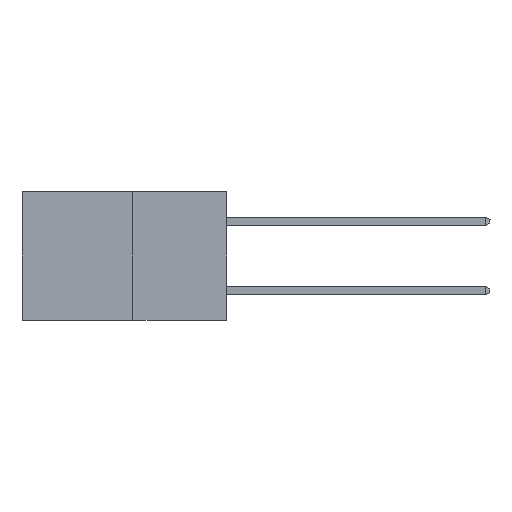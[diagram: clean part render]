
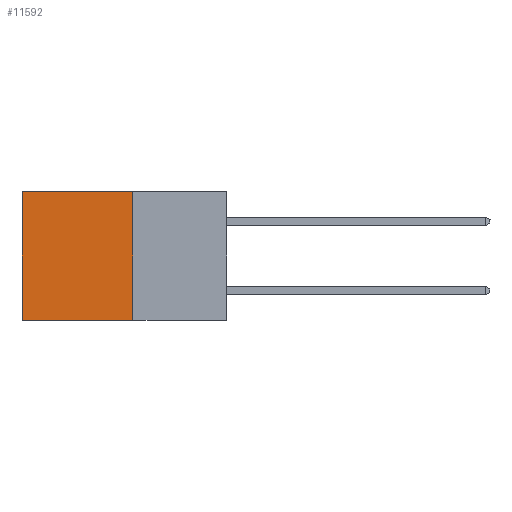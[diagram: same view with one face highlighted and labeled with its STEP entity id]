
A CAD part, left-side view. The second image highlights one B-rep face of the part: STEP entity #11592.
In plain terms, the highlighted planar face has unit normal (-1, 0, 0).
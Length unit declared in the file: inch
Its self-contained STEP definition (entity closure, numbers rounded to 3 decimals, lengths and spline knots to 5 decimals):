
#15 = LINE ( 'NONE', #7952, #9856 ) ;
#1263 = ORIENTED_EDGE ( 'NONE', *, *, #12215, .T. ) ;
#1660 = PLANE ( 'NONE',  #14526 ) ;
#1710 = DIRECTION ( 'NONE',  ( 1., 0., 0. ) ) ;
#2517 = FACE_OUTER_BOUND ( 'NONE', #6134, .T. ) ;
#3730 = VERTEX_POINT ( 'NONE', #15855 ) ;
#3775 = VECTOR ( 'NONE', #7048, 39.37008 ) ;
#3787 = VERTEX_POINT ( 'NONE', #13471 ) ;
#3988 = EDGE_CURVE ( 'NONE', #3787, #5481, #15, .T. ) ;
#5089 = LINE ( 'NONE', #5234, #7692 ) ;
#5234 = CARTESIAN_POINT ( 'NONE',  ( 0.277, 0.27, 0. ) ) ;
#5241 = EDGE_CURVE ( 'NONE', #11155, #3730, #7139, .T. ) ;
#5481 = VERTEX_POINT ( 'NONE', #13715 ) ;
#5519 = VECTOR ( 'NONE', #9380, 39.37008 ) ;
#6134 = EDGE_LOOP ( 'NONE', ( #10816, #13954, #7459, #1263 ) ) ;
#6419 = EDGE_CURVE ( 'NONE', #3730, #5481, #12318, .T. ) ;
#7048 = DIRECTION ( 'NONE',  ( 0., 0., -1. ) ) ;
#7139 = LINE ( 'NONE', #13351, #3775 ) ;
#7459 = ORIENTED_EDGE ( 'NONE', *, *, #5241, .F. ) ;
#7692 = VECTOR ( 'NONE', #12852, 39.37008 ) ;
#7813 = DIRECTION ( 'NONE',  ( 0., 0., -1. ) ) ;
#7952 = CARTESIAN_POINT ( 'NONE',  ( 0.277, 0.59, -0.37 ) ) ;
#9380 = DIRECTION ( 'NONE',  ( 0., 1., 0. ) ) ;
#9856 = VECTOR ( 'NONE', #7813, 39.37008 ) ;
#10660 = DIRECTION ( 'NONE',  ( 0., 0., -1. ) ) ;
#10816 = ORIENTED_EDGE ( 'NONE', *, *, #3988, .T. ) ;
#11155 = VERTEX_POINT ( 'NONE', #15951 ) ;
#11592 = ADVANCED_FACE ( 'NONE', ( #2517 ), #1660, .F. ) ;
#12215 = EDGE_CURVE ( 'NONE', #11155, #3787, #5089, .T. ) ;
#12318 = LINE ( 'NONE', #15499, #5519 ) ;
#12852 = DIRECTION ( 'NONE',  ( 0., 1., 0. ) ) ;
#13021 = CARTESIAN_POINT ( 'NONE',  ( 0.277, 0.27, -0.37 ) ) ;
#13351 = CARTESIAN_POINT ( 'NONE',  ( 0.277, 0.27, -0.37 ) ) ;
#13471 = CARTESIAN_POINT ( 'NONE',  ( 0.277, 0.59, 0. ) ) ;
#13715 = CARTESIAN_POINT ( 'NONE',  ( 0.277, 0.59, -0.37 ) ) ;
#13954 = ORIENTED_EDGE ( 'NONE', *, *, #6419, .F. ) ;
#14526 = AXIS2_PLACEMENT_3D ( 'NONE', #13021, #1710, #10660 ) ;
#15499 = CARTESIAN_POINT ( 'NONE',  ( 0.277, 0.27, -0.37 ) ) ;
#15855 = CARTESIAN_POINT ( 'NONE',  ( 0.277, 0.27, -0.37 ) ) ;
#15951 = CARTESIAN_POINT ( 'NONE',  ( 0.277, 0.27, 0. ) ) ;
